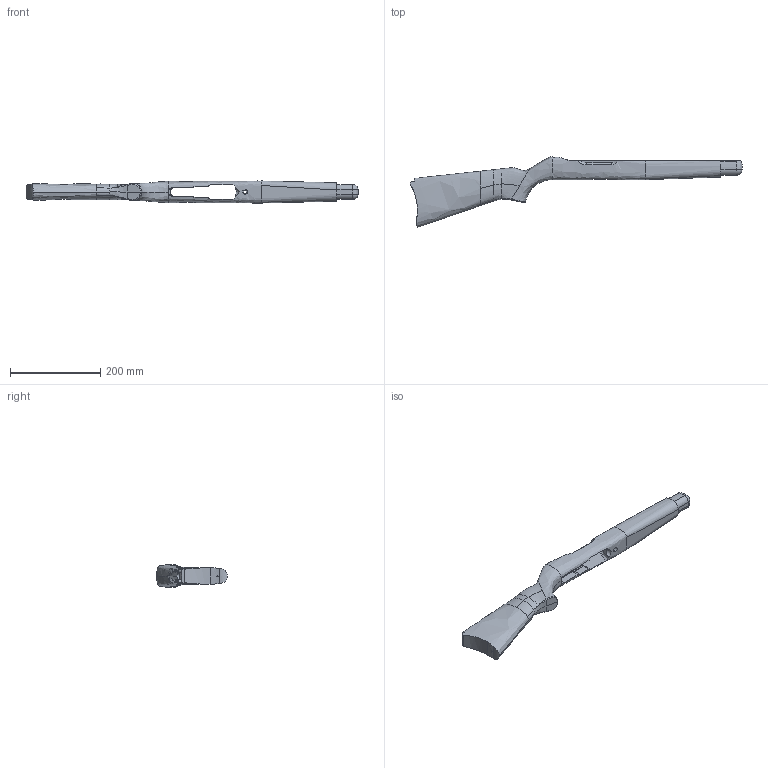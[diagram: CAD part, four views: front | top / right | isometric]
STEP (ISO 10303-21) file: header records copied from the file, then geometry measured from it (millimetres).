
FILE_DESCRIPTION (( 'STEP AP214' ), '1' );
FILE_NAME ('41 Stock.IGS_sldprt.STEP', '2024-01-06T03:12:40', ( '' ), ( '' ), 'SwSTEP 2.0', 'SolidWorks 2021', '' );
FILE_SCHEMA (( 'AUTOMOTIVE_DESIGN' ));
Length unit declared in the file: millimetre
Products named in the file (1): 41 Stock.IGS_sldprt
Bounding box: 737.16 x 156.84 x 49 mm (x, y, z)
Volume: 1211418.8 mm3; surface area: 143069.4 mm2
Topology: 1 solids, 1 shells, 142 faces, 398 edges, 251 vertices
Faces by surface type: cylinder 48, plane 41, bspline 39, sphere 5, torus 5, cone 4
Entity records: 18425 total; most frequent: CARTESIAN_POINT 15199, ORIENTED_EDGE 780, DIRECTION 499, EDGE_CURVE 390, VERTEX_POINT 251, AXIS2_PLACEMENT_3D 182, B_SPLINE_CURVE_WITH_KNOTS 169, EDGE_LOOP 147
